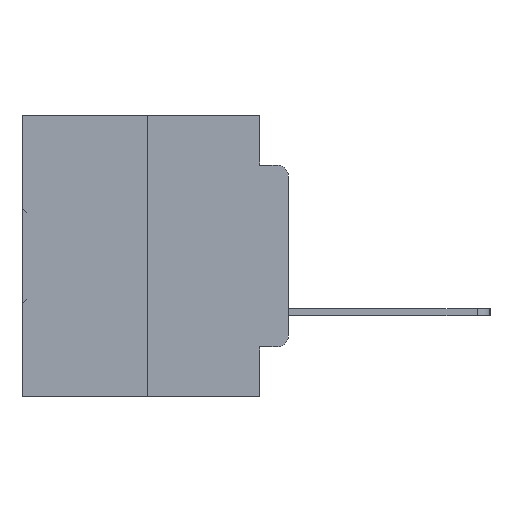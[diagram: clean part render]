
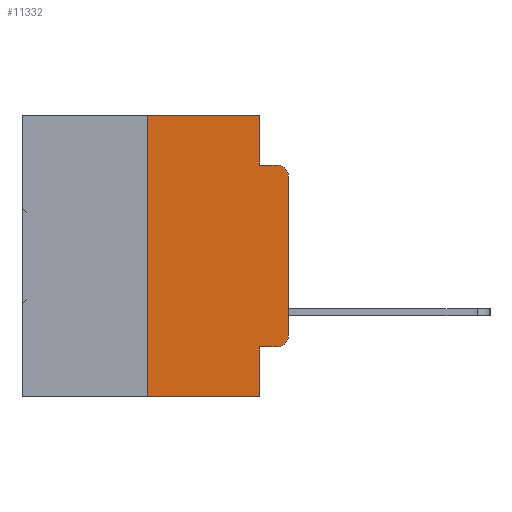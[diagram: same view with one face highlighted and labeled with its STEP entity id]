
A CAD part, left-side view. The second image highlights one B-rep face of the part: STEP entity #11332.
In plain terms, the highlighted planar face has unit normal (-1, 0, 0).
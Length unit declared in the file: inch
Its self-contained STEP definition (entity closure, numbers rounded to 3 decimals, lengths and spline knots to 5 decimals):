
#132 = ORIENTED_EDGE ( 'NONE', *, *, #18603, .T. ) ;
#583 = ORIENTED_EDGE ( 'NONE', *, *, #3460, .T. ) ;
#655 = FACE_OUTER_BOUND ( 'NONE', #21225, .T. ) ;
#736 = EDGE_CURVE ( 'NONE', #22373, #11603, #32540, .T. ) ;
#1153 = DIRECTION ( 'NONE',  ( -1., 0., 0. ) ) ;
#2174 = DIRECTION ( 'NONE',  ( 0., -1., 0. ) ) ;
#3087 = DIRECTION ( 'NONE',  ( 0., 0., -1. ) ) ;
#3271 = PLANE ( 'NONE',  #32223 ) ;
#3460 = EDGE_CURVE ( 'NONE', #21249, #23509, #5712, .T. ) ;
#4360 = DIRECTION ( 'NONE',  ( -1., 0., 0. ) ) ;
#5712 = CIRCLE ( 'NONE', #22994, 0.02 ) ;
#6712 = CARTESIAN_POINT ( 'NONE',  ( 0., 0.051, 0. ) ) ;
#7125 = DIRECTION ( 'NONE',  ( 0., 0., -1. ) ) ;
#7188 = DIRECTION ( 'NONE',  ( 0., -1., 0. ) ) ;
#7275 = ORIENTED_EDGE ( 'NONE', *, *, #10737, .F. ) ;
#7522 = LINE ( 'NONE', #27769, #13548 ) ;
#7552 = VECTOR ( 'NONE', #15906, 39.37008 ) ;
#7634 = CARTESIAN_POINT ( 'NONE',  ( 0., 0.051, -0.5 ) ) ;
#7676 = CARTESIAN_POINT ( 'NONE',  ( 0., 0.02, -0.4115 ) ) ;
#7837 = VECTOR ( 'NONE', #28301, 39.37008 ) ;
#8123 = ORIENTED_EDGE ( 'NONE', *, *, #21509, .F. ) ;
#8485 = CARTESIAN_POINT ( 'NONE',  ( 0., 0.473, 0. ) ) ;
#8600 = LINE ( 'NONE', #30640, #14612 ) ;
#8639 = LINE ( 'NONE', #18107, #7837 ) ;
#9028 = VERTEX_POINT ( 'NONE', #13065 ) ;
#9038 = VERTEX_POINT ( 'NONE', #10489 ) ;
#9709 = ORIENTED_EDGE ( 'NONE', *, *, #736, .F. ) ;
#10489 = CARTESIAN_POINT ( 'NONE',  ( 0., 0.051, -0.4115 ) ) ;
#10519 = ORIENTED_EDGE ( 'NONE', *, *, #28766, .T. ) ;
#10737 = EDGE_CURVE ( 'NONE', #12426, #9028, #8639, .T. ) ;
#11156 = DIRECTION ( 'NONE',  ( 1., 0., 0. ) ) ;
#11332 = ADVANCED_FACE ( 'NONE', ( #655 ), #3271, .F. ) ;
#11603 = VERTEX_POINT ( 'NONE', #6712 ) ;
#11628 = VECTOR ( 'NONE', #7188, 39.37008 ) ;
#11883 = CARTESIAN_POINT ( 'NONE',  ( 0., 0., -0.3915 ) ) ;
#12196 = VECTOR ( 'NONE', #29292, 39.37008 ) ;
#12426 = VERTEX_POINT ( 'NONE', #24591 ) ;
#13065 = CARTESIAN_POINT ( 'NONE',  ( 0., 0.02, -0.0885 ) ) ;
#13314 = CARTESIAN_POINT ( 'NONE',  ( 0., 0.25, 0. ) ) ;
#13548 = VECTOR ( 'NONE', #2174, 39.37008 ) ;
#13741 = ORIENTED_EDGE ( 'NONE', *, *, #15646, .T. ) ;
#14025 = VERTEX_POINT ( 'NONE', #25633 ) ;
#14612 = VECTOR ( 'NONE', #25471, 39.37008 ) ;
#15646 = EDGE_CURVE ( 'NONE', #9038, #21249, #32310, .T. ) ;
#15906 = DIRECTION ( 'NONE',  ( 0., 0., 1. ) ) ;
#16774 = CARTESIAN_POINT ( 'NONE',  ( 0., 0.02, -0.1085 ) ) ;
#17302 = CARTESIAN_POINT ( 'NONE',  ( 0., 0.051, 0. ) ) ;
#17530 = VERTEX_POINT ( 'NONE', #27159 ) ;
#18107 = CARTESIAN_POINT ( 'NONE',  ( 0., 0.051, -0.0885 ) ) ;
#18182 = VERTEX_POINT ( 'NONE', #7634 ) ;
#18368 = EDGE_CURVE ( 'NONE', #9038, #18182, #30789, .T. ) ;
#18603 = EDGE_CURVE ( 'NONE', #14025, #9028, #25268, .T. ) ;
#18861 = ORIENTED_EDGE ( 'NONE', *, *, #18368, .F. ) ;
#19257 = DIRECTION ( 'NONE',  ( 0., 0., -1. ) ) ;
#19499 = LINE ( 'NONE', #17302, #25445 ) ;
#19711 = CARTESIAN_POINT ( 'NONE',  ( 0., 0.02, -0.3915 ) ) ;
#20003 = ORIENTED_EDGE ( 'NONE', *, *, #31439, .T. ) ;
#21225 = EDGE_LOOP ( 'NONE', ( #20003, #132, #7275, #8123, #9709, #29896, #10519, #18861, #13741, #583 ) ) ;
#21249 = VERTEX_POINT ( 'NONE', #7676 ) ;
#21509 = EDGE_CURVE ( 'NONE', #11603, #12426, #19499, .T. ) ;
#21741 = CARTESIAN_POINT ( 'NONE',  ( 0., 0.051, -0.4115 ) ) ;
#22255 = DIRECTION ( 'NONE',  ( 0., 0., -1. ) ) ;
#22373 = VERTEX_POINT ( 'NONE', #30596 ) ;
#22994 = AXIS2_PLACEMENT_3D ( 'NONE', #19711, #4360, #22255 ) ;
#23509 = VERTEX_POINT ( 'NONE', #11883 ) ;
#24099 = VECTOR ( 'NONE', #3087, 39.37008 ) ;
#24591 = CARTESIAN_POINT ( 'NONE',  ( 0., 0.051, -0.0885 ) ) ;
#24974 = CARTESIAN_POINT ( 'NONE',  ( 0., 0.473, 0. ) ) ;
#25268 = CIRCLE ( 'NONE', #26727, 0.02 ) ;
#25445 = VECTOR ( 'NONE', #7125, 39.37008 ) ;
#25471 = DIRECTION ( 'NONE',  ( 0., 0., 1. ) ) ;
#25550 = EDGE_CURVE ( 'NONE', #17530, #22373, #27817, .T. ) ;
#25633 = CARTESIAN_POINT ( 'NONE',  ( 0., 0., -0.1085 ) ) ;
#26727 = AXIS2_PLACEMENT_3D ( 'NONE', #16774, #1153, #19257 ) ;
#27159 = CARTESIAN_POINT ( 'NONE',  ( 0., 0.25, -0.5 ) ) ;
#27769 = CARTESIAN_POINT ( 'NONE',  ( 0., 0.473, -0.5 ) ) ;
#27817 = LINE ( 'NONE', #13314, #7552 ) ;
#28301 = DIRECTION ( 'NONE',  ( 0., -1., 0. ) ) ;
#28766 = EDGE_CURVE ( 'NONE', #17530, #18182, #7522, .T. ) ;
#28874 = DIRECTION ( 'NONE',  ( 0., 0., -1. ) ) ;
#29292 = DIRECTION ( 'NONE',  ( 0., -1., 0. ) ) ;
#29896 = ORIENTED_EDGE ( 'NONE', *, *, #25550, .F. ) ;
#30596 = CARTESIAN_POINT ( 'NONE',  ( 0., 0.25, 0. ) ) ;
#30640 = CARTESIAN_POINT ( 'NONE',  ( 0., 0., 0. ) ) ;
#30789 = LINE ( 'NONE', #31060, #24099 ) ;
#31060 = CARTESIAN_POINT ( 'NONE',  ( 0., 0.051, 0. ) ) ;
#31439 = EDGE_CURVE ( 'NONE', #23509, #14025, #8600, .T. ) ;
#32223 = AXIS2_PLACEMENT_3D ( 'NONE', #8485, #11156, #28874 ) ;
#32310 = LINE ( 'NONE', #21741, #12196 ) ;
#32540 = LINE ( 'NONE', #24974, #11628 ) ;
